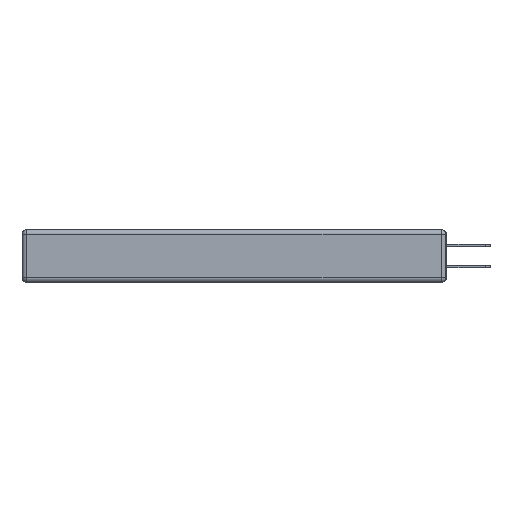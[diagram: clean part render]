
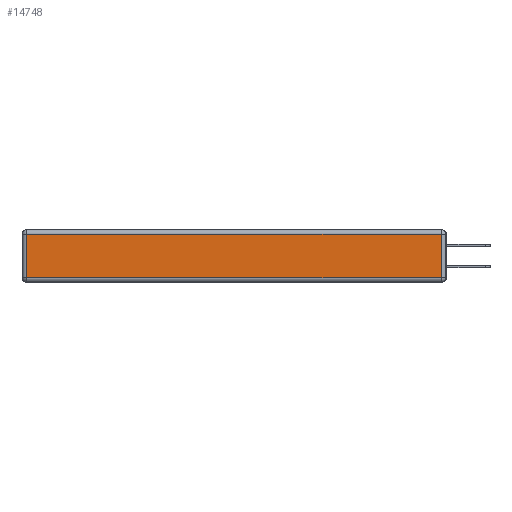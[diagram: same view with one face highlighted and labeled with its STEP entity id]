
A CAD part, left-side view. The second image highlights one B-rep face of the part: STEP entity #14748.
In plain terms, the highlighted planar face has unit normal (-1, 0, 0).
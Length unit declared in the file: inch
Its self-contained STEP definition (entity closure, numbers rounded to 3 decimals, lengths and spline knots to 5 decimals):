
#891 = VERTEX_POINT ( 'NONE', #13093 ) ;
#1444 = DIRECTION ( 'NONE',  ( 0., 1., 0. ) ) ;
#1826 = CARTESIAN_POINT ( 'NONE',  ( 0., 0., -0.313 ) ) ;
#2525 = VERTEX_POINT ( 'NONE', #3475 ) ;
#3329 = CARTESIAN_POINT ( 'NONE',  ( 0., 2.72, -0.03 ) ) ;
#3475 = CARTESIAN_POINT ( 'NONE',  ( 0., 0.03, -0.313 ) ) ;
#3785 = LINE ( 'NONE', #14278, #4037 ) ;
#3867 = ORIENTED_EDGE ( 'NONE', *, *, #9317, .T. ) ;
#4037 = VECTOR ( 'NONE', #9079, 39.37008 ) ;
#4639 = CARTESIAN_POINT ( 'NONE',  ( 0., 0.03, -0.03 ) ) ;
#5025 = DIRECTION ( 'NONE',  ( 0., 0., 1. ) ) ;
#7698 = VECTOR ( 'NONE', #1444, 39.37008 ) ;
#9079 = DIRECTION ( 'NONE',  ( 0., 0., 1. ) ) ;
#9317 = EDGE_CURVE ( 'NONE', #16509, #891, #12104, .T. ) ;
#11747 = PLANE ( 'NONE',  #18312 ) ;
#11783 = LINE ( 'NONE', #13285, #7698 ) ;
#11863 = VERTEX_POINT ( 'NONE', #4639 ) ;
#11896 = DIRECTION ( 'NONE',  ( -1., 0., 0. ) ) ;
#12104 = LINE ( 'NONE', #15439, #17418 ) ;
#12178 = DIRECTION ( 'NONE',  ( 0., 0., -1. ) ) ;
#13093 = CARTESIAN_POINT ( 'NONE',  ( 0., 2.72, -0.313 ) ) ;
#13285 = CARTESIAN_POINT ( 'NONE',  ( 0., 2.75, -0.03 ) ) ;
#13790 = ORIENTED_EDGE ( 'NONE', *, *, #21835, .T. ) ;
#13917 = VECTOR ( 'NONE', #18815, 39.37008 ) ;
#14278 = CARTESIAN_POINT ( 'NONE',  ( 0., 0.03, -0.343 ) ) ;
#14748 = ADVANCED_FACE ( 'NONE', ( #18125 ), #11747, .T. ) ;
#15439 = CARTESIAN_POINT ( 'NONE',  ( 0., 2.72, -0.343 ) ) ;
#16136 = ORIENTED_EDGE ( 'NONE', *, *, #17488, .T. ) ;
#16194 = EDGE_LOOP ( 'NONE', ( #18893, #13790, #16136, #3867 ) ) ;
#16509 = VERTEX_POINT ( 'NONE', #3329 ) ;
#17418 = VECTOR ( 'NONE', #12178, 39.37008 ) ;
#17488 = EDGE_CURVE ( 'NONE', #11863, #16509, #11783, .T. ) ;
#17644 = EDGE_CURVE ( 'NONE', #891, #2525, #21415, .T. ) ;
#18125 = FACE_OUTER_BOUND ( 'NONE', #16194, .T. ) ;
#18312 = AXIS2_PLACEMENT_3D ( 'NONE', #22146, #11896, #5025 ) ;
#18815 = DIRECTION ( 'NONE',  ( 0., -1., 0. ) ) ;
#18893 = ORIENTED_EDGE ( 'NONE', *, *, #17644, .T. ) ;
#21415 = LINE ( 'NONE', #1826, #13917 ) ;
#21835 = EDGE_CURVE ( 'NONE', #2525, #11863, #3785, .T. ) ;
#22146 = CARTESIAN_POINT ( 'NONE',  ( 0., 0., -0.343 ) ) ;
